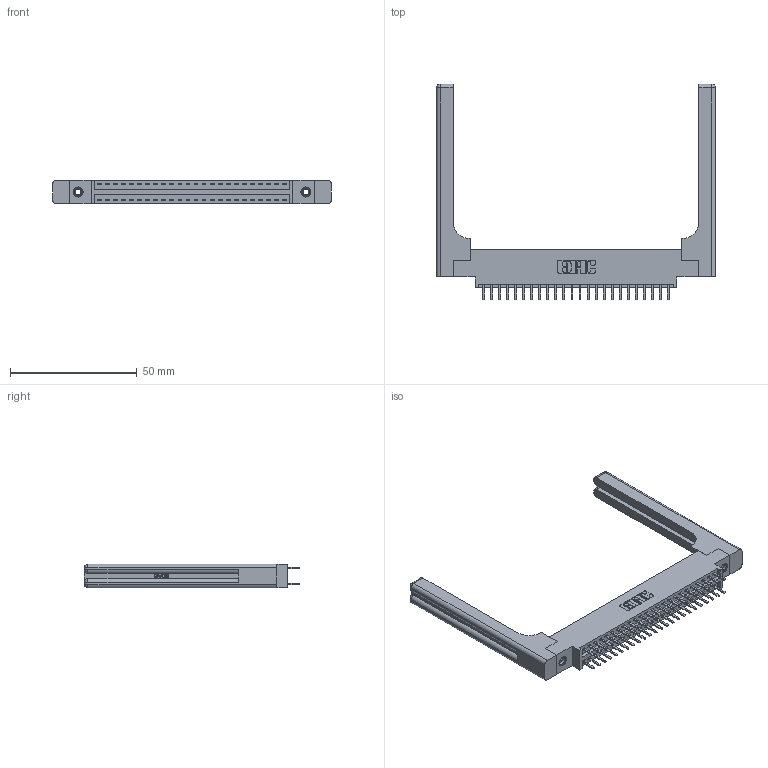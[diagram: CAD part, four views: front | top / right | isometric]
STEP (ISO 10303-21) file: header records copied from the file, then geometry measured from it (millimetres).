
FILE_DESCRIPTION (( 'STEP AP203' ), '1' );
FILE_NAME ('396-048-520-858.STEP', '2019-11-02T06:54:06', ( '' ), ( '' ), 'SwSTEP 2.0', 'SolidWorks 2016', '' );
FILE_SCHEMA (( 'CONFIG_CONTROL_DESIGN' ));
Length unit declared in the file: inch
Products named in the file (5): 346 Part_0.170 Offset - 0.156 Dia-TH; 345-292-001_345-293-120; 345-250-001_345-250-001-102; 346-220-058_345-220-058; 396-048-520-858
Assembly tree (53 placements, depth 2):
  396-048-520-858
    346 Part_0.170 Offset - 0.156 Dia-TH
    345-292-001_345-293-120  x48
    345-250-001_345-250-001-102  x2
    346-220-058_345-220-058  x2
Bounding box: 110.26 x 85.29 x 9.4 mm (x, y, z)
Volume: 17930.6 mm3; surface area: 19165.5 mm2
Topology: 53 solids, 53 shells, 3070 faces, 8831 edges, 5738 vertices
Faces by surface type: plane 2004, cylinder 1006, bspline 36, cone 12, sphere 8, torus 4
Entity records: 23514 total; most frequent: CARTESIAN_POINT 4921, ORIENTED_EDGE 3640, DIRECTION 3308, EDGE_CURVE 1820, VECTOR 1496, LINE 1496, VERTEX_POINT 1202, AXIS2_PLACEMENT_3D 906
